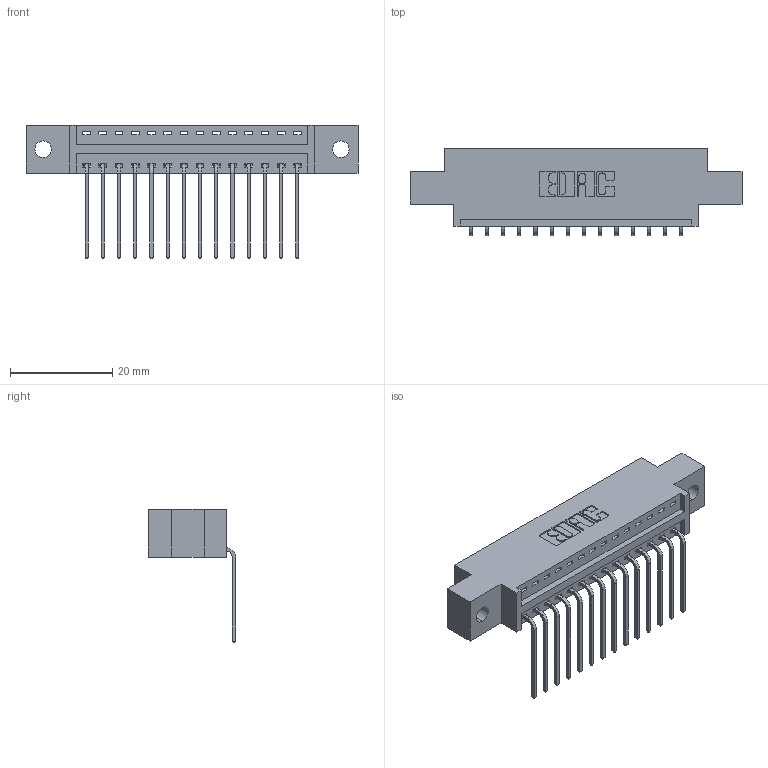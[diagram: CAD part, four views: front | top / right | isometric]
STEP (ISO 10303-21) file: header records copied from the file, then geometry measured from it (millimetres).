
FILE_DESCRIPTION (( 'STEP AP203' ), '1' );
FILE_NAME ('396-014-559-602.STEP', '2018-08-31T11:16:00', ( '' ), ( '' ), 'SwSTEP 2.0', 'SolidWorks 2016', '' );
FILE_SCHEMA (( 'CONFIG_CONTROL_DESIGN' ));
Length unit declared in the file: inch
Products named in the file (3): 345-292-001_558 559 Tail - 1; 396-014-559-602; 346 Part_0.170 Offset - 0.128 Dia
Assembly tree (15 placements, depth 2):
  396-014-559-602
    346 Part_0.170 Offset - 0.128 Dia
    345-292-001_558 559 Tail - 1  x14
Bounding box: 65.02 x 17.08 x 26.16 mm (x, y, z)
Volume: 5886.7 mm3; surface area: 7222.8 mm2
Topology: 15 solids, 15 shells, 966 faces, 2889 edges, 1906 vertices
Faces by surface type: plane 668, cylinder 298
Entity records: 12677 total; most frequent: CARTESIAN_POINT 2190, ORIENTED_EDGE 2138, DIRECTION 1965, EDGE_CURVE 1069, LINE 881, VECTOR 881, VERTEX_POINT 710, AXIS2_PLACEMENT_3D 542
